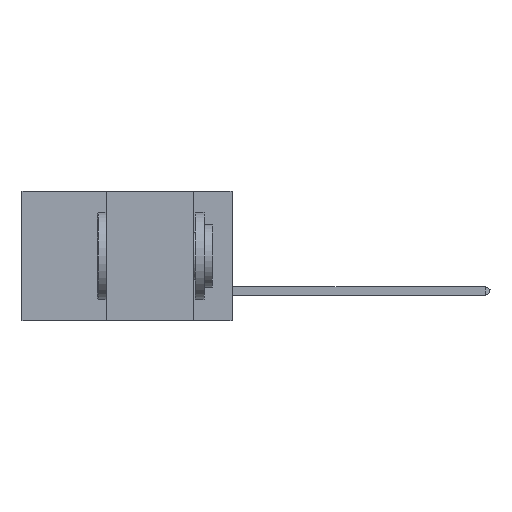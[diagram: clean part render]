
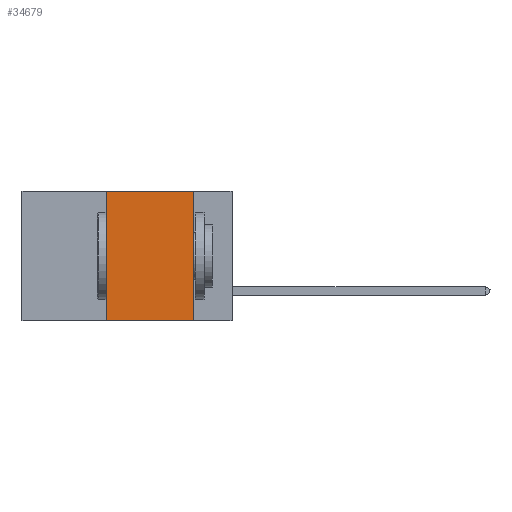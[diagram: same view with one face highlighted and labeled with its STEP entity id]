
A CAD part, left-side view. The second image highlights one B-rep face of the part: STEP entity #34679.
In plain terms, the highlighted planar face has unit normal (-1, 0, 0).
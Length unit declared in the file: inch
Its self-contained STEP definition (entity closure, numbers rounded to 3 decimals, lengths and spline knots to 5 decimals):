
#2048 = CARTESIAN_POINT ( 'NONE',  ( 0., 0.36, -0.37 ) ) ;
#2925 = ORIENTED_EDGE ( 'NONE', *, *, #26798, .T. ) ;
#4553 = DIRECTION ( 'NONE',  ( 1., 0., 0. ) ) ;
#5422 = DIRECTION ( 'NONE',  ( 0., 0., -1. ) ) ;
#5592 = CARTESIAN_POINT ( 'NONE',  ( 0., 0.11, -0.37 ) ) ;
#6168 = ORIENTED_EDGE ( 'NONE', *, *, #33544, .F. ) ;
#6456 = VECTOR ( 'NONE', #38404, 39.37008 ) ;
#6908 = VECTOR ( 'NONE', #32364, 39.37008 ) ;
#7223 = EDGE_CURVE ( 'NONE', #22850, #23833, #9924, .T. ) ;
#9924 = LINE ( 'NONE', #22667, #18779 ) ;
#10622 = CARTESIAN_POINT ( 'NONE',  ( 0., 0.6, 0. ) ) ;
#11262 = FACE_OUTER_BOUND ( 'NONE', #30521, .T. ) ;
#11770 = CARTESIAN_POINT ( 'NONE',  ( 0., 0.11, 0. ) ) ;
#12080 = ORIENTED_EDGE ( 'NONE', *, *, #7223, .F. ) ;
#13745 = CARTESIAN_POINT ( 'NONE',  ( 0., 0.36, 0. ) ) ;
#14240 = LINE ( 'NONE', #34872, #6456 ) ;
#16648 = ORIENTED_EDGE ( 'NONE', *, *, #17687, .F. ) ;
#17687 = EDGE_CURVE ( 'NONE', #33598, #22850, #22082, .T. ) ;
#18779 = VECTOR ( 'NONE', #5422, 39.37008 ) ;
#21124 = AXIS2_PLACEMENT_3D ( 'NONE', #31002, #4553, #39536 ) ;
#22082 = LINE ( 'NONE', #10622, #6908 ) ;
#22667 = CARTESIAN_POINT ( 'NONE',  ( 0., 0.11, 0. ) ) ;
#22850 = VERTEX_POINT ( 'NONE', #11770 ) ;
#23116 = DIRECTION ( 'NONE',  ( 0., 0., 1. ) ) ;
#23345 = VECTOR ( 'NONE', #23116, 39.37008 ) ;
#23833 = VERTEX_POINT ( 'NONE', #5592 ) ;
#25444 = LINE ( 'NONE', #39408, #23345 ) ;
#26798 = EDGE_CURVE ( 'NONE', #38436, #23833, #14240, .T. ) ;
#27595 = PLANE ( 'NONE',  #21124 ) ;
#30521 = EDGE_LOOP ( 'NONE', ( #12080, #16648, #6168, #2925 ) ) ;
#31002 = CARTESIAN_POINT ( 'NONE',  ( 0., 0.6, 0. ) ) ;
#32364 = DIRECTION ( 'NONE',  ( 0., -1., 0. ) ) ;
#33544 = EDGE_CURVE ( 'NONE', #38436, #33598, #25444, .T. ) ;
#33598 = VERTEX_POINT ( 'NONE', #13745 ) ;
#34679 = ADVANCED_FACE ( 'NONE', ( #11262 ), #27595, .F. ) ;
#34872 = CARTESIAN_POINT ( 'NONE',  ( 0., 0.6, -0.37 ) ) ;
#38404 = DIRECTION ( 'NONE',  ( 0., -1., 0. ) ) ;
#38436 = VERTEX_POINT ( 'NONE', #2048 ) ;
#39408 = CARTESIAN_POINT ( 'NONE',  ( 0., 0.36, 0. ) ) ;
#39536 = DIRECTION ( 'NONE',  ( 0., 0., -1. ) ) ;
